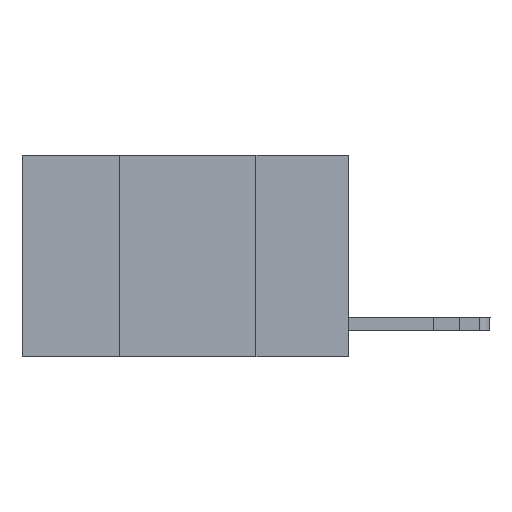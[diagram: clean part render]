
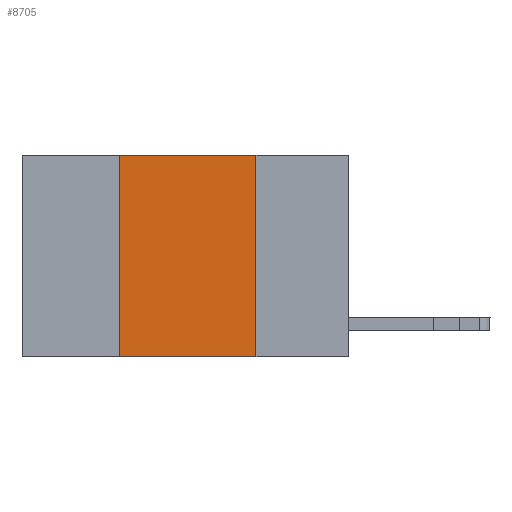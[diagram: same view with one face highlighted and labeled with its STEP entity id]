
A CAD part, left-side view. The second image highlights one B-rep face of the part: STEP entity #8705.
In plain terms, the highlighted planar face has unit normal (-1, 0, 0).
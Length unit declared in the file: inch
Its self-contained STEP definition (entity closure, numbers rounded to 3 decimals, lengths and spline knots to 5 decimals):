
#51 = PLANE ( 'NONE',  #1287 ) ;
#495 = VERTEX_POINT ( 'NONE', #6555 ) ;
#1287 = AXIS2_PLACEMENT_3D ( 'NONE', #9773, #5554, #10694 ) ;
#1649 = VECTOR ( 'NONE', #8796, 39.37008 ) ;
#1987 = CARTESIAN_POINT ( 'NONE',  ( 0., 0.6, 0. ) ) ;
#2140 = EDGE_LOOP ( 'NONE', ( #5078, #5728, #12043, #11546 ) ) ;
#2450 = CARTESIAN_POINT ( 'NONE',  ( 0., 0.17, 0. ) ) ;
#2687 = EDGE_CURVE ( 'NONE', #495, #8917, #4115, .T. ) ;
#2716 = CARTESIAN_POINT ( 'NONE',  ( 0., 0.17, -0.37 ) ) ;
#4115 = LINE ( 'NONE', #1987, #9609 ) ;
#4752 = CARTESIAN_POINT ( 'NONE',  ( 0., 0.6, -0.37 ) ) ;
#4775 = VERTEX_POINT ( 'NONE', #2716 ) ;
#4818 = DIRECTION ( 'NONE',  ( 0., -1., 0. ) ) ;
#5078 = ORIENTED_EDGE ( 'NONE', *, *, #8777, .F. ) ;
#5547 = LINE ( 'NONE', #9834, #1649 ) ;
#5554 = DIRECTION ( 'NONE',  ( 1., 0., 0. ) ) ;
#5728 = ORIENTED_EDGE ( 'NONE', *, *, #2687, .F. ) ;
#5928 = EDGE_CURVE ( 'NONE', #9988, #495, #5547, .T. ) ;
#6024 = VECTOR ( 'NONE', #8662, 39.37008 ) ;
#6079 = LINE ( 'NONE', #4752, #8019 ) ;
#6555 = CARTESIAN_POINT ( 'NONE',  ( 0., 0.42, 0. ) ) ;
#8019 = VECTOR ( 'NONE', #4818, 39.37008 ) ;
#8596 = LINE ( 'NONE', #11956, #6024 ) ;
#8662 = DIRECTION ( 'NONE',  ( 0., 0., -1. ) ) ;
#8705 = ADVANCED_FACE ( 'NONE', ( #10629 ), #51, .F. ) ;
#8777 = EDGE_CURVE ( 'NONE', #8917, #4775, #8596, .T. ) ;
#8796 = DIRECTION ( 'NONE',  ( 0., 0., 1. ) ) ;
#8917 = VERTEX_POINT ( 'NONE', #2450 ) ;
#9609 = VECTOR ( 'NONE', #11836, 39.37008 ) ;
#9773 = CARTESIAN_POINT ( 'NONE',  ( 0., 0.6, 0. ) ) ;
#9834 = CARTESIAN_POINT ( 'NONE',  ( 0., 0.42, 0. ) ) ;
#9988 = VERTEX_POINT ( 'NONE', #12024 ) ;
#10629 = FACE_OUTER_BOUND ( 'NONE', #2140, .T. ) ;
#10694 = DIRECTION ( 'NONE',  ( 0., 0., -1. ) ) ;
#11546 = ORIENTED_EDGE ( 'NONE', *, *, #13046, .T. ) ;
#11836 = DIRECTION ( 'NONE',  ( 0., -1., 0. ) ) ;
#11956 = CARTESIAN_POINT ( 'NONE',  ( 0., 0.17, 0. ) ) ;
#12024 = CARTESIAN_POINT ( 'NONE',  ( 0., 0.42, -0.37 ) ) ;
#12043 = ORIENTED_EDGE ( 'NONE', *, *, #5928, .F. ) ;
#13046 = EDGE_CURVE ( 'NONE', #9988, #4775, #6079, .T. ) ;
